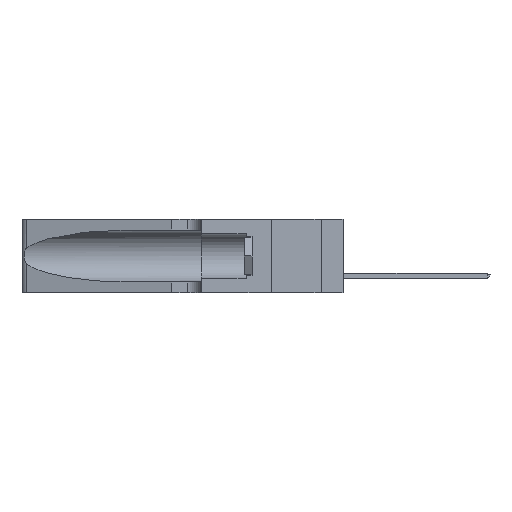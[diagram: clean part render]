
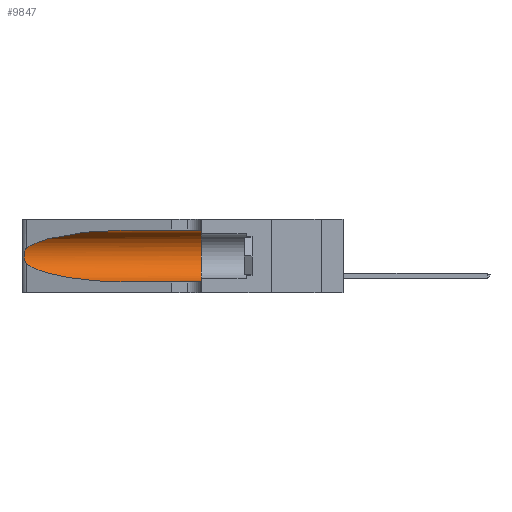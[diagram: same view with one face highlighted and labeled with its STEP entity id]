
A CAD part, left-side view. The second image highlights one B-rep face of the part: STEP entity #9847.
In plain terms, the highlighted cylindrical face has radius 3.308 mm (diameter 6.617 mm), a partial arc.
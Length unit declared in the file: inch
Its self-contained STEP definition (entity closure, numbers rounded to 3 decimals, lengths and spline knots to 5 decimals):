
#164 = ORIENTED_EDGE ( 'NONE', *, *, #37889, .T. ) ;
#1637 = DIRECTION ( 'NONE',  ( 0., 1., 0. ) ) ;
#3060 = AXIS2_PLACEMENT_3D ( 'NONE', #10536, #1637, #22863 ) ;
#3445 = CARTESIAN_POINT ( 'NONE',  ( 0.25487, 1.22718, 0.22369 ) ) ;
#3574 = CARTESIAN_POINT ( 'NONE',  ( 0.1305, 0.72297, 0.31525 ) ) ;
#4315 = CARTESIAN_POINT ( 'NONE',  ( 0.25487, 1.22718, 0.22369 ) ) ;
#4843 = CARTESIAN_POINT ( 'NONE',  ( 0.25854, 1.2359, 0.20912 ) ) ;
#4948 = B_SPLINE_CURVE_WITH_KNOTS ( 'NONE', 3,
 ( #4315, #16404, #19581, #7770, #4843, #26000, #34639, #16667, #19717, #22733, #32527, #8035, #23399, #26542 ),
 .UNSPECIFIED., .F., .F.,
 ( 4, 2, 2, 2, 2, 2, 4 ),
 ( 0., 0.00027, 0.00053, 0.00107, 0.0016, 0.00187, 0.00214 ),
 .UNSPECIFIED. ) ;
#5546 = VERTEX_POINT ( 'NONE', #38144 ) ;
#6801 = CARTESIAN_POINT ( 'NONE',  ( 0.2373, 1.15595, 0.28018 ) ) ;
#7061 = CARTESIAN_POINT ( 'NONE',  ( 0.18966, 0.96281, 0.31525 ) ) ;
#7213 = VERTEX_POINT ( 'NONE', #10590 ) ;
#7770 = CARTESIAN_POINT ( 'NONE',  ( 0.25787, 1.23484, 0.2124 ) ) ;
#8035 = CARTESIAN_POINT ( 'NONE',  ( 0.25639, 1.23186, 0.15144 ) ) ;
#8058 = CARTESIAN_POINT ( 'NONE',  ( 0.1305, 0.72297, 0.05475 ) ) ;
#9014 = EDGE_CURVE ( 'NONE', #24737, #27230, #13269, .T. ) ;
#9171 = ORIENTED_EDGE ( 'NONE', *, *, #17614, .T. ) ;
#9847 = ADVANCED_FACE ( 'NONE', ( #37351 ), #36857, .F. ) ;
#10536 = CARTESIAN_POINT ( 'NONE',  ( 0.1305, 0.35, 0.185 ) ) ;
#10590 = CARTESIAN_POINT ( 'NONE',  ( 0.1305, 0.72297, 0.31525 ) ) ;
#12547 = ORIENTED_EDGE ( 'NONE', *, *, #9014, .T. ) ;
#12753 = CARTESIAN_POINT ( 'NONE',  ( 0.18966, 0.96281, 0.05475 ) ) ;
#13269 = LINE ( 'NONE', #37132, #33171 ) ;
#13419 = VERTEX_POINT ( 'NONE', #23517 ) ;
#13530 = DIRECTION ( 'NONE',  ( 0., -1., 0. ) ) ;
#14243 = CARTESIAN_POINT ( 'NONE',  ( 0.1305, 0.35, 0.05475 ) ) ;
#14405 = VECTOR ( 'NONE', #13530, 39.37008 ) ;
#15302 = ORIENTED_EDGE ( 'NONE', *, *, #20927, .T. ) ;
#16104 = ORIENTED_EDGE ( 'NONE', *, *, #22227, .F. ) ;
#16404 = CARTESIAN_POINT ( 'NONE',  ( 0.25555, 1.22994, 0.2215 ) ) ;
#16667 = CARTESIAN_POINT ( 'NONE',  ( 0.26075, 1.23896, 0.178 ) ) ;
#16715 = AXIS2_PLACEMENT_3D ( 'NONE', #34775, #38095, #23003 ) ;
#17614 = EDGE_CURVE ( 'NONE', #7213, #34434, #26036, .T. ) ;
#19581 = CARTESIAN_POINT ( 'NONE',  ( 0.25639, 1.23184, 0.21858 ) ) ;
#19717 = CARTESIAN_POINT ( 'NONE',  ( 0.26017, 1.23833, 0.17102 ) ) ;
#20927 = EDGE_CURVE ( 'NONE', #5546, #24737, #21270, .T. ) ;
#21270 =( BOUNDED_CURVE ( )  B_SPLINE_CURVE ( 3, ( #30863, #34064, #12753, #22294 ),
 .UNSPECIFIED., .F., .F. ) 
 B_SPLINE_CURVE_WITH_KNOTS ( ( 4, 4 ),
 ( 3.44316, 4.71239 ),
 .UNSPECIFIED. ) 
 CURVE ( )  GEOMETRIC_REPRESENTATION_ITEM ( )  RATIONAL_B_SPLINE_CURVE ( ( 1., 0.87, 0.87, 1. ) ) 
 REPRESENTATION_ITEM ( '' )  );
#21329 = CIRCLE ( 'NONE', #3060, 0.13025 ) ;
#21499 = LINE ( 'NONE', #25921, #14405 ) ;
#21660 = DIRECTION ( 'NONE',  ( 0., -1., 0. ) ) ;
#22227 = EDGE_CURVE ( 'NONE', #13419, #27230, #21329, .T. ) ;
#22294 = CARTESIAN_POINT ( 'NONE',  ( 0.1305, 0.72297, 0.05475 ) ) ;
#22733 = CARTESIAN_POINT ( 'NONE',  ( 0.25856, 1.23593, 0.16098 ) ) ;
#22863 = DIRECTION ( 'NONE',  ( 0., 0., 1. ) ) ;
#23003 = DIRECTION ( 'NONE',  ( 0., 0., -1. ) ) ;
#23399 = CARTESIAN_POINT ( 'NONE',  ( 0.25555, 1.22993, 0.14849 ) ) ;
#23517 = CARTESIAN_POINT ( 'NONE',  ( 0.1305, 0.35, 0.31525 ) ) ;
#24737 = VERTEX_POINT ( 'NONE', #8058 ) ;
#25921 = CARTESIAN_POINT ( 'NONE',  ( 0.1305, 1.61858, 0.31525 ) ) ;
#26000 = CARTESIAN_POINT ( 'NONE',  ( 0.26018, 1.23835, 0.19895 ) ) ;
#26036 =( BOUNDED_CURVE ( )  B_SPLINE_CURVE ( 3, ( #3574, #7061, #6801, #3445 ),
 .UNSPECIFIED., .F., .F. ) 
 B_SPLINE_CURVE_WITH_KNOTS ( ( 4, 4 ),
 ( 1.5708, 2.84003 ),
 .UNSPECIFIED. ) 
 CURVE ( )  GEOMETRIC_REPRESENTATION_ITEM ( )  RATIONAL_B_SPLINE_CURVE ( ( 1., 0.87, 0.87, 1. ) ) 
 REPRESENTATION_ITEM ( '' )  );
#26542 = CARTESIAN_POINT ( 'NONE',  ( 0.25487, 1.22718, 0.14631 ) ) ;
#27230 = VERTEX_POINT ( 'NONE', #14243 ) ;
#28850 = EDGE_LOOP ( 'NONE', ( #9171, #164, #15302, #12547, #16104, #31303 ) ) ;
#30863 = CARTESIAN_POINT ( 'NONE',  ( 0.25487, 1.22718, 0.14631 ) ) ;
#31303 = ORIENTED_EDGE ( 'NONE', *, *, #34102, .F. ) ;
#32527 = CARTESIAN_POINT ( 'NONE',  ( 0.25789, 1.23486, 0.15765 ) ) ;
#33171 = VECTOR ( 'NONE', #21660, 39.37008 ) ;
#34064 = CARTESIAN_POINT ( 'NONE',  ( 0.2373, 1.15595, 0.08982 ) ) ;
#34102 = EDGE_CURVE ( 'NONE', #7213, #13419, #21499, .T. ) ;
#34434 = VERTEX_POINT ( 'NONE', #38820 ) ;
#34639 = CARTESIAN_POINT ( 'NONE',  ( 0.26075, 1.23896, 0.19203 ) ) ;
#34775 = CARTESIAN_POINT ( 'NONE',  ( 0.1305, 1.61858, 0.185 ) ) ;
#36857 = CYLINDRICAL_SURFACE ( 'NONE', #16715, 0.13025 ) ;
#37132 = CARTESIAN_POINT ( 'NONE',  ( 0.1305, 1.61858, 0.05475 ) ) ;
#37351 = FACE_OUTER_BOUND ( 'NONE', #28850, .T. ) ;
#37889 = EDGE_CURVE ( 'NONE', #34434, #5546, #4948, .T. ) ;
#38095 = DIRECTION ( 'NONE',  ( 0., -1., 0. ) ) ;
#38144 = CARTESIAN_POINT ( 'NONE',  ( 0.25487, 1.22718, 0.14631 ) ) ;
#38820 = CARTESIAN_POINT ( 'NONE',  ( 0.25487, 1.22718, 0.22369 ) ) ;
